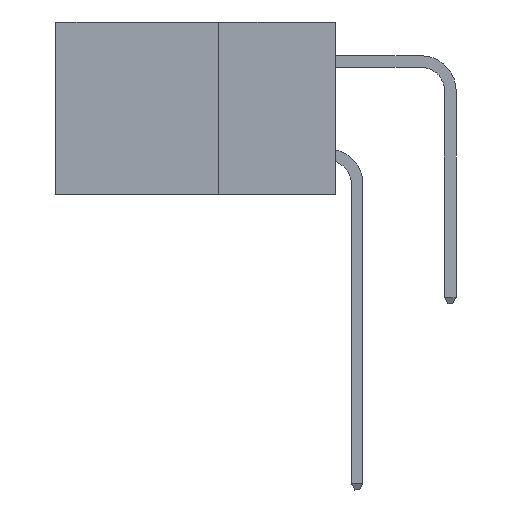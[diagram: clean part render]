
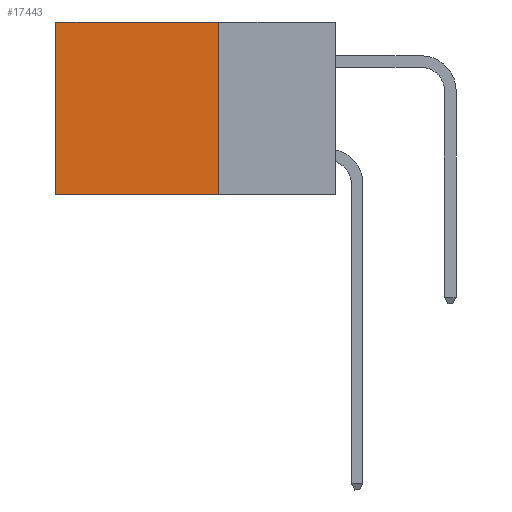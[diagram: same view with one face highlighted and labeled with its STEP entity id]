
A CAD part, left-side view. The second image highlights one B-rep face of the part: STEP entity #17443.
In plain terms, the highlighted planar face has unit normal (-1, 0, 0).
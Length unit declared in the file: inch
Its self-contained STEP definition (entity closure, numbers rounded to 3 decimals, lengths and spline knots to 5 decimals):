
#836 = VERTEX_POINT ( 'NONE', #21084 ) ;
#2127 = DIRECTION ( 'NONE',  ( 0., 0., -1. ) ) ;
#2628 = VECTOR ( 'NONE', #2127, 39.37008 ) ;
#4170 = CARTESIAN_POINT ( 'NONE',  ( 0.2875, 0.6, 0. ) ) ;
#4492 = LINE ( 'NONE', #16213, #19903 ) ;
#5342 = EDGE_CURVE ( 'NONE', #12076, #836, #4492, .T. ) ;
#6318 = DIRECTION ( 'NONE',  ( 0., 0., -1. ) ) ;
#6812 = AXIS2_PLACEMENT_3D ( 'NONE', #6993, #15190, #7588 ) ;
#6993 = CARTESIAN_POINT ( 'NONE',  ( 0.2875, 0.25, 0. ) ) ;
#7588 = DIRECTION ( 'NONE',  ( 0., 0., -1. ) ) ;
#8645 = EDGE_LOOP ( 'NONE', ( #8960, #22272, #24422, #16343 ) ) ;
#8651 = VERTEX_POINT ( 'NONE', #9606 ) ;
#8960 = ORIENTED_EDGE ( 'NONE', *, *, #5342, .T. ) ;
#9606 = CARTESIAN_POINT ( 'NONE',  ( 0.2875, 0.25, 0. ) ) ;
#9880 = CARTESIAN_POINT ( 'NONE',  ( 0.2875, 0.25, 0. ) ) ;
#11069 = LINE ( 'NONE', #21277, #19909 ) ;
#12076 = VERTEX_POINT ( 'NONE', #4170 ) ;
#12234 = FACE_OUTER_BOUND ( 'NONE', #8645, .T. ) ;
#13148 = PLANE ( 'NONE',  #6812 ) ;
#13202 = CARTESIAN_POINT ( 'NONE',  ( 0.2875, 0.25, -0.37 ) ) ;
#14166 = CARTESIAN_POINT ( 'NONE',  ( 0.2875, 0.25, 0. ) ) ;
#14661 = VECTOR ( 'NONE', #24485, 39.37008 ) ;
#15190 = DIRECTION ( 'NONE',  ( 1., 0., 0. ) ) ;
#16213 = CARTESIAN_POINT ( 'NONE',  ( 0.2875, 0.6, 0. ) ) ;
#16343 = ORIENTED_EDGE ( 'NONE', *, *, #23431, .T. ) ;
#17443 = ADVANCED_FACE ( 'NONE', ( #12234 ), #13148, .F. ) ;
#18682 = LINE ( 'NONE', #9880, #2628 ) ;
#19903 = VECTOR ( 'NONE', #6318, 39.37008 ) ;
#19909 = VECTOR ( 'NONE', #23287, 39.37008 ) ;
#20973 = LINE ( 'NONE', #14166, #14661 ) ;
#21084 = CARTESIAN_POINT ( 'NONE',  ( 0.2875, 0.6, -0.37 ) ) ;
#21277 = CARTESIAN_POINT ( 'NONE',  ( 0.2875, 0.25, -0.37 ) ) ;
#22272 = ORIENTED_EDGE ( 'NONE', *, *, #25636, .F. ) ;
#23013 = VERTEX_POINT ( 'NONE', #13202 ) ;
#23287 = DIRECTION ( 'NONE',  ( 0., 1., 0. ) ) ;
#23431 = EDGE_CURVE ( 'NONE', #8651, #12076, #20973, .T. ) ;
#24422 = ORIENTED_EDGE ( 'NONE', *, *, #25276, .F. ) ;
#24485 = DIRECTION ( 'NONE',  ( 0., 1., 0. ) ) ;
#25276 = EDGE_CURVE ( 'NONE', #8651, #23013, #18682, .T. ) ;
#25636 = EDGE_CURVE ( 'NONE', #23013, #836, #11069, .T. ) ;
